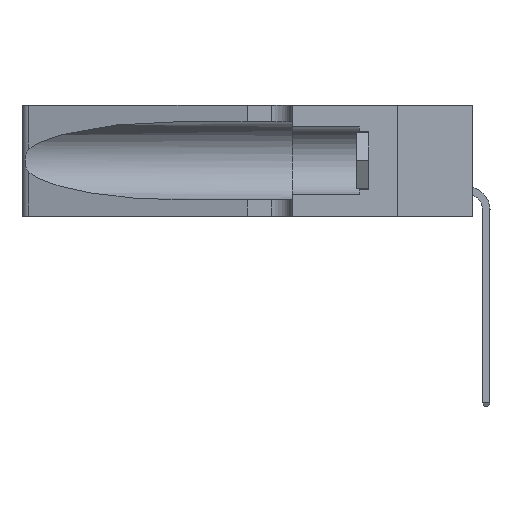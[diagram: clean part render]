
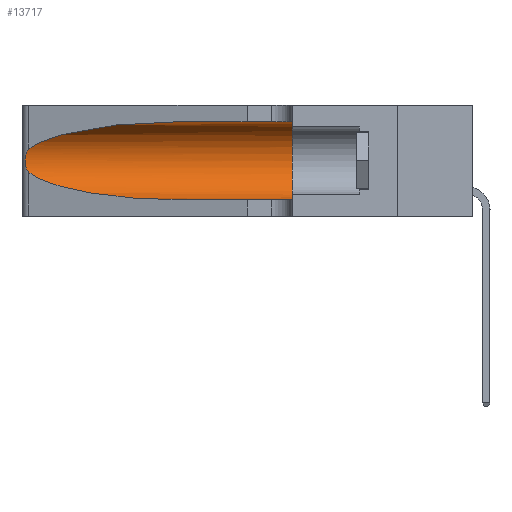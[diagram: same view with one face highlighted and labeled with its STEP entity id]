
A CAD part, left-side view. The second image highlights one B-rep face of the part: STEP entity #13717.
In plain terms, the highlighted cylindrical face has radius 3.308 mm (diameter 6.617 mm), a partial arc.
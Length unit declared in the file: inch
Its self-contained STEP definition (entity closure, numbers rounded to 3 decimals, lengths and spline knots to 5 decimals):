
#359 = CARTESIAN_POINT ( 'NONE',  ( 0.25487, 1.22718, 0.14631 ) ) ;
#2017 = ORIENTED_EDGE ( 'NONE', *, *, #27506, .F. ) ;
#2364 = EDGE_LOOP ( 'NONE', ( #9575, #13325, #19448, #13127, #10475, #2017 ) ) ;
#2767 = AXIS2_PLACEMENT_3D ( 'NONE', #5075, #17292, #3624 ) ;
#2780 = B_SPLINE_CURVE_WITH_KNOTS ( 'NONE', 3,
 ( #17348, #17523, #23863, #4728, #19668, #21809, #9038, #23761, #23588, #21425, #15116, #13167, #23959, #359 ),
 .UNSPECIFIED., .F., .F.,
 ( 4, 2, 2, 2, 2, 2, 4 ),
 ( 0., 0.00027, 0.00053, 0.00107, 0.0016, 0.00187, 0.00214 ),
 .UNSPECIFIED. ) ;
#2907 = FACE_OUTER_BOUND ( 'NONE', #2364, .T. ) ;
#3073 = CARTESIAN_POINT ( 'NONE',  ( 0.1305, 0.35, 0.185 ) ) ;
#3556 = CYLINDRICAL_SURFACE ( 'NONE', #2767, 0.13025 ) ;
#3624 = DIRECTION ( 'NONE',  ( 0., 0., -1. ) ) ;
#4399 = CARTESIAN_POINT ( 'NONE',  ( 0.2373, 1.15595, 0.08982 ) ) ;
#4728 = CARTESIAN_POINT ( 'NONE',  ( 0.25787, 1.23484, 0.2124 ) ) ;
#5042 = EDGE_CURVE ( 'NONE', #11954, #8273, #17657, .T. ) ;
#5075 = CARTESIAN_POINT ( 'NONE',  ( 0.1305, 1.61858, 0.185 ) ) ;
#5730 = CARTESIAN_POINT ( 'NONE',  ( 0.1305, 1.61858, 0.05475 ) ) ;
#7212 = CARTESIAN_POINT ( 'NONE',  ( 0.1305, 0.35, 0.05475 ) ) ;
#7221 = CARTESIAN_POINT ( 'NONE',  ( 0.1305, 0.72297, 0.05475 ) ) ;
#7359 = DIRECTION ( 'NONE',  ( 0., 1., 0. ) ) ;
#7544 = VERTEX_POINT ( 'NONE', #7212 ) ;
#8273 = VERTEX_POINT ( 'NONE', #18647 ) ;
#8832 = EDGE_CURVE ( 'NONE', #21503, #7544, #21337, .T. ) ;
#9038 = CARTESIAN_POINT ( 'NONE',  ( 0.26075, 1.23896, 0.19203 ) ) ;
#9575 = ORIENTED_EDGE ( 'NONE', *, *, #5042, .T. ) ;
#10080 = DIRECTION ( 'NONE',  ( 0., -1., 0. ) ) ;
#10475 = ORIENTED_EDGE ( 'NONE', *, *, #17823, .F. ) ;
#11621 = CARTESIAN_POINT ( 'NONE',  ( 0.2373, 1.15595, 0.28018 ) ) ;
#11717 = CARTESIAN_POINT ( 'NONE',  ( 0.1305, 0.72297, 0.31525 ) ) ;
#11954 = VERTEX_POINT ( 'NONE', #18059 ) ;
#13127 = ORIENTED_EDGE ( 'NONE', *, *, #8832, .T. ) ;
#13167 = CARTESIAN_POINT ( 'NONE',  ( 0.25639, 1.23186, 0.15144 ) ) ;
#13325 = ORIENTED_EDGE ( 'NONE', *, *, #24596, .T. ) ;
#13333 = VERTEX_POINT ( 'NONE', #15889 ) ;
#13334 = VECTOR ( 'NONE', #19627, 39.37008 ) ;
#13685 = CARTESIAN_POINT ( 'NONE',  ( 0.1305, 1.61858, 0.31525 ) ) ;
#13717 = ADVANCED_FACE ( 'NONE', ( #2907 ), #3556, .F. ) ;
#14708 = CIRCLE ( 'NONE', #27488, 0.13025 ) ;
#15116 = CARTESIAN_POINT ( 'NONE',  ( 0.25789, 1.23486, 0.15765 ) ) ;
#15721 = VECTOR ( 'NONE', #10080, 39.37008 ) ;
#15889 = CARTESIAN_POINT ( 'NONE',  ( 0.1305, 0.35, 0.31525 ) ) ;
#16005 = EDGE_CURVE ( 'NONE', #18152, #21503, #26378, .T. ) ;
#17292 = DIRECTION ( 'NONE',  ( 0., -1., 0. ) ) ;
#17348 = CARTESIAN_POINT ( 'NONE',  ( 0.25487, 1.22718, 0.22369 ) ) ;
#17523 = CARTESIAN_POINT ( 'NONE',  ( 0.25555, 1.22994, 0.2215 ) ) ;
#17657 =( BOUNDED_CURVE ( )  B_SPLINE_CURVE ( 3, ( #11717, #24708, #11621, #26603 ),
 .UNSPECIFIED., .F., .F. ) 
 B_SPLINE_CURVE_WITH_KNOTS ( ( 4, 4 ),
 ( 1.5708, 2.84003 ),
 .UNSPECIFIED. ) 
 CURVE ( )  GEOMETRIC_REPRESENTATION_ITEM ( )  RATIONAL_B_SPLINE_CURVE ( ( 1., 0.87, 0.87, 1. ) ) 
 REPRESENTATION_ITEM ( '' )  );
#17823 = EDGE_CURVE ( 'NONE', #13333, #7544, #14708, .T. ) ;
#17856 = CARTESIAN_POINT ( 'NONE',  ( 0.18966, 0.96281, 0.05475 ) ) ;
#18059 = CARTESIAN_POINT ( 'NONE',  ( 0.1305, 0.72297, 0.31525 ) ) ;
#18080 = DIRECTION ( 'NONE',  ( 0., 0., 1. ) ) ;
#18152 = VERTEX_POINT ( 'NONE', #19442 ) ;
#18636 = LINE ( 'NONE', #13685, #13334 ) ;
#18647 = CARTESIAN_POINT ( 'NONE',  ( 0.25487, 1.22718, 0.22369 ) ) ;
#19442 = CARTESIAN_POINT ( 'NONE',  ( 0.25487, 1.22718, 0.14631 ) ) ;
#19448 = ORIENTED_EDGE ( 'NONE', *, *, #16005, .T. ) ;
#19627 = DIRECTION ( 'NONE',  ( 0., -1., 0. ) ) ;
#19668 = CARTESIAN_POINT ( 'NONE',  ( 0.25854, 1.2359, 0.20912 ) ) ;
#21337 = LINE ( 'NONE', #5730, #15721 ) ;
#21425 = CARTESIAN_POINT ( 'NONE',  ( 0.25856, 1.23593, 0.16098 ) ) ;
#21503 = VERTEX_POINT ( 'NONE', #27005 ) ;
#21809 = CARTESIAN_POINT ( 'NONE',  ( 0.26018, 1.23835, 0.19895 ) ) ;
#22144 = CARTESIAN_POINT ( 'NONE',  ( 0.25487, 1.22718, 0.14631 ) ) ;
#23588 = CARTESIAN_POINT ( 'NONE',  ( 0.26017, 1.23833, 0.17102 ) ) ;
#23761 = CARTESIAN_POINT ( 'NONE',  ( 0.26075, 1.23896, 0.178 ) ) ;
#23863 = CARTESIAN_POINT ( 'NONE',  ( 0.25639, 1.23184, 0.21858 ) ) ;
#23959 = CARTESIAN_POINT ( 'NONE',  ( 0.25555, 1.22993, 0.14849 ) ) ;
#24596 = EDGE_CURVE ( 'NONE', #8273, #18152, #2780, .T. ) ;
#24708 = CARTESIAN_POINT ( 'NONE',  ( 0.18966, 0.96281, 0.31525 ) ) ;
#26378 =( BOUNDED_CURVE ( )  B_SPLINE_CURVE ( 3, ( #22144, #4399, #17856, #7221 ),
 .UNSPECIFIED., .F., .T. ) 
 B_SPLINE_CURVE_WITH_KNOTS ( ( 4, 4 ),
 ( 3.44316, 4.71239 ),
 .UNSPECIFIED. ) 
 CURVE ( )  GEOMETRIC_REPRESENTATION_ITEM ( )  RATIONAL_B_SPLINE_CURVE ( ( 1., 0.87, 0.87, 1. ) ) 
 REPRESENTATION_ITEM ( '' )  );
#26603 = CARTESIAN_POINT ( 'NONE',  ( 0.25487, 1.22718, 0.22369 ) ) ;
#27005 = CARTESIAN_POINT ( 'NONE',  ( 0.1305, 0.72297, 0.05475 ) ) ;
#27488 = AXIS2_PLACEMENT_3D ( 'NONE', #3073, #7359, #18080 ) ;
#27506 = EDGE_CURVE ( 'NONE', #11954, #13333, #18636, .T. ) ;
